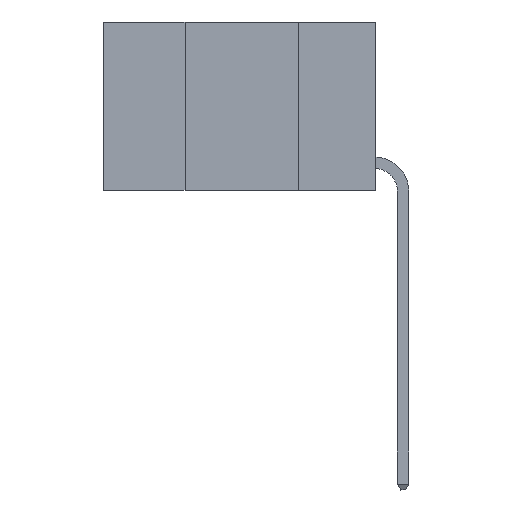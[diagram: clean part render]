
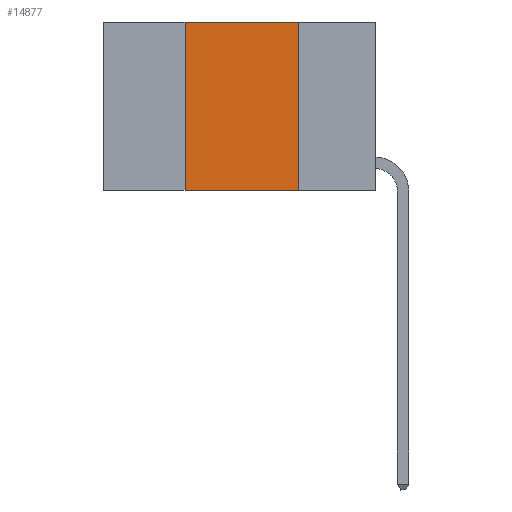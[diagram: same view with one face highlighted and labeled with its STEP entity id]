
A CAD part, left-side view. The second image highlights one B-rep face of the part: STEP entity #14877.
In plain terms, the highlighted planar face has unit normal (-1, 0, 0).
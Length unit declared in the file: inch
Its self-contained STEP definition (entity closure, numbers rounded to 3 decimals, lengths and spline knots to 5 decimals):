
#1166 = ORIENTED_EDGE ( 'NONE', *, *, #5878, .F. ) ;
#1261 = LINE ( 'NONE', #7952, #3965 ) ;
#1366 = ORIENTED_EDGE ( 'NONE', *, *, #15058, .F. ) ;
#1464 = DIRECTION ( 'NONE',  ( 0., -1., 0. ) ) ;
#2187 = VECTOR ( 'NONE', #9823, 39.37008 ) ;
#2631 = VERTEX_POINT ( 'NONE', #5157 ) ;
#2675 = EDGE_LOOP ( 'NONE', ( #7292, #1166, #1366, #14848 ) ) ;
#3038 = CARTESIAN_POINT ( 'NONE',  ( 0., 0.17, -0.37 ) ) ;
#3292 = VERTEX_POINT ( 'NONE', #3038 ) ;
#3965 = VECTOR ( 'NONE', #12953, 39.37008 ) ;
#4107 = DIRECTION ( 'NONE',  ( 0., 0., -1. ) ) ;
#5053 = AXIS2_PLACEMENT_3D ( 'NONE', #9234, #13539, #4107 ) ;
#5157 = CARTESIAN_POINT ( 'NONE',  ( 0., 0.42, -0.37 ) ) ;
#5487 = PLANE ( 'NONE',  #5053 ) ;
#5621 = VECTOR ( 'NONE', #1464, 39.37008 ) ;
#5656 = LINE ( 'NONE', #12558, #2187 ) ;
#5878 = EDGE_CURVE ( 'NONE', #10987, #8476, #14816, .T. ) ;
#7292 = ORIENTED_EDGE ( 'NONE', *, *, #15953, .F. ) ;
#7918 = FACE_OUTER_BOUND ( 'NONE', #2675, .T. ) ;
#7952 = CARTESIAN_POINT ( 'NONE',  ( 0., 0.17, 0. ) ) ;
#8476 = VERTEX_POINT ( 'NONE', #12461 ) ;
#8510 = LINE ( 'NONE', #9660, #10605 ) ;
#9234 = CARTESIAN_POINT ( 'NONE',  ( 0., 0.6, 0. ) ) ;
#9660 = CARTESIAN_POINT ( 'NONE',  ( 0., 0.42, 0. ) ) ;
#9662 = EDGE_CURVE ( 'NONE', #2631, #3292, #5656, .T. ) ;
#9823 = DIRECTION ( 'NONE',  ( 0., -1., 0. ) ) ;
#10002 = DIRECTION ( 'NONE',  ( 0., 0., 1. ) ) ;
#10568 = CARTESIAN_POINT ( 'NONE',  ( 0., 0.42, 0. ) ) ;
#10605 = VECTOR ( 'NONE', #10002, 39.37008 ) ;
#10987 = VERTEX_POINT ( 'NONE', #10568 ) ;
#12185 = CARTESIAN_POINT ( 'NONE',  ( 0., 0.6, 0. ) ) ;
#12461 = CARTESIAN_POINT ( 'NONE',  ( 0., 0.17, 0. ) ) ;
#12558 = CARTESIAN_POINT ( 'NONE',  ( 0., 0.6, -0.37 ) ) ;
#12953 = DIRECTION ( 'NONE',  ( 0., 0., -1. ) ) ;
#13539 = DIRECTION ( 'NONE',  ( 1., 0., 0. ) ) ;
#14816 = LINE ( 'NONE', #12185, #5621 ) ;
#14848 = ORIENTED_EDGE ( 'NONE', *, *, #9662, .T. ) ;
#14877 = ADVANCED_FACE ( 'NONE', ( #7918 ), #5487, .F. ) ;
#15058 = EDGE_CURVE ( 'NONE', #2631, #10987, #8510, .T. ) ;
#15953 = EDGE_CURVE ( 'NONE', #8476, #3292, #1261, .T. ) ;
